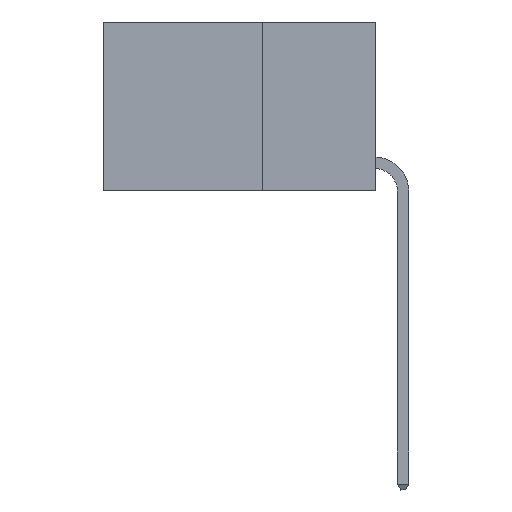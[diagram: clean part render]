
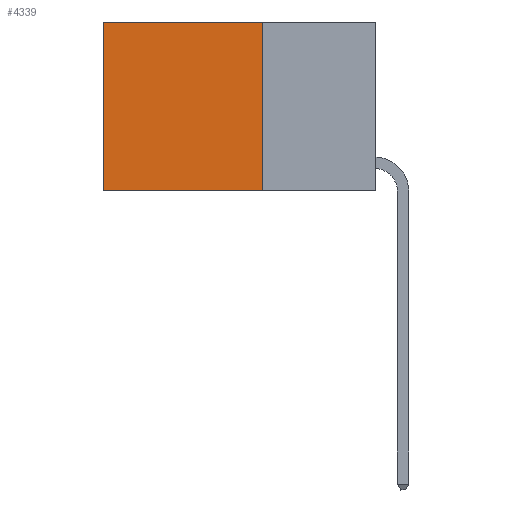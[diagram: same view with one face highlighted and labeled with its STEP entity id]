
A CAD part, left-side view. The second image highlights one B-rep face of the part: STEP entity #4339.
In plain terms, the highlighted planar face has unit normal (-1, 0, 0).
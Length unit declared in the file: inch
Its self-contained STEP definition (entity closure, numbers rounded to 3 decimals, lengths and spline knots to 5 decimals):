
#25 = DIRECTION ( 'NONE',  ( 0., 1., 0. ) ) ;
#79 = DIRECTION ( 'NONE',  ( 1., 0., 0. ) ) ;
#1170 = EDGE_CURVE ( 'NONE', #15205, #9643, #11654, .T. ) ;
#2304 = DIRECTION ( 'NONE',  ( 0., 0., -1. ) ) ;
#2839 = VECTOR ( 'NONE', #25, 39.37008 ) ;
#3019 = VERTEX_POINT ( 'NONE', #3702 ) ;
#3134 = CARTESIAN_POINT ( 'NONE',  ( 0.2625, 0.6, -0.37 ) ) ;
#3306 = EDGE_CURVE ( 'NONE', #3019, #15258, #9256, .T. ) ;
#3702 = CARTESIAN_POINT ( 'NONE',  ( 0.2625, 0.25, 0. ) ) ;
#4141 = AXIS2_PLACEMENT_3D ( 'NONE', #13239, #79, #4872 ) ;
#4339 = ADVANCED_FACE ( 'NONE', ( #10913 ), #5022, .F. ) ;
#4872 = DIRECTION ( 'NONE',  ( 0., 0., -1. ) ) ;
#5003 = CARTESIAN_POINT ( 'NONE',  ( 0.2625, 0.25, 0. ) ) ;
#5022 = PLANE ( 'NONE',  #4141 ) ;
#5141 = CARTESIAN_POINT ( 'NONE',  ( 0.2625, 0.25, -0.37 ) ) ;
#6011 = VECTOR ( 'NONE', #2304, 39.37008 ) ;
#6134 = ORIENTED_EDGE ( 'NONE', *, *, #3306, .F. ) ;
#6891 = DIRECTION ( 'NONE',  ( 0., 0., -1. ) ) ;
#8509 = EDGE_CURVE ( 'NONE', #15258, #9643, #9674, .T. ) ;
#8861 = ORIENTED_EDGE ( 'NONE', *, *, #1170, .T. ) ;
#9256 = LINE ( 'NONE', #14079, #14794 ) ;
#9643 = VERTEX_POINT ( 'NONE', #3134 ) ;
#9674 = LINE ( 'NONE', #11949, #2839 ) ;
#9697 = ORIENTED_EDGE ( 'NONE', *, *, #8509, .F. ) ;
#9873 = DIRECTION ( 'NONE',  ( 0., 1., 0. ) ) ;
#10913 = FACE_OUTER_BOUND ( 'NONE', #12058, .T. ) ;
#11654 = LINE ( 'NONE', #15070, #6011 ) ;
#11949 = CARTESIAN_POINT ( 'NONE',  ( 0.2625, 0.25, -0.37 ) ) ;
#12058 = EDGE_LOOP ( 'NONE', ( #8861, #9697, #6134, #15077 ) ) ;
#12133 = LINE ( 'NONE', #5003, #13811 ) ;
#13239 = CARTESIAN_POINT ( 'NONE',  ( 0.2625, 0.25, 0. ) ) ;
#13274 = CARTESIAN_POINT ( 'NONE',  ( 0.2625, 0.6, 0. ) ) ;
#13811 = VECTOR ( 'NONE', #9873, 39.37008 ) ;
#14079 = CARTESIAN_POINT ( 'NONE',  ( 0.2625, 0.25, 0. ) ) ;
#14650 = EDGE_CURVE ( 'NONE', #3019, #15205, #12133, .T. ) ;
#14794 = VECTOR ( 'NONE', #6891, 39.37008 ) ;
#15070 = CARTESIAN_POINT ( 'NONE',  ( 0.2625, 0.6, 0. ) ) ;
#15077 = ORIENTED_EDGE ( 'NONE', *, *, #14650, .T. ) ;
#15205 = VERTEX_POINT ( 'NONE', #13274 ) ;
#15258 = VERTEX_POINT ( 'NONE', #5141 ) ;
